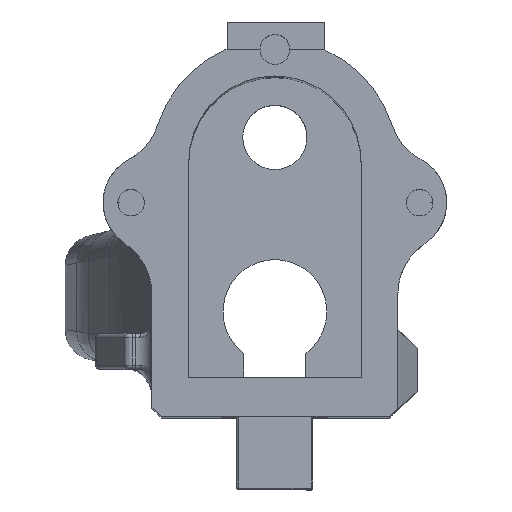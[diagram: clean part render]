
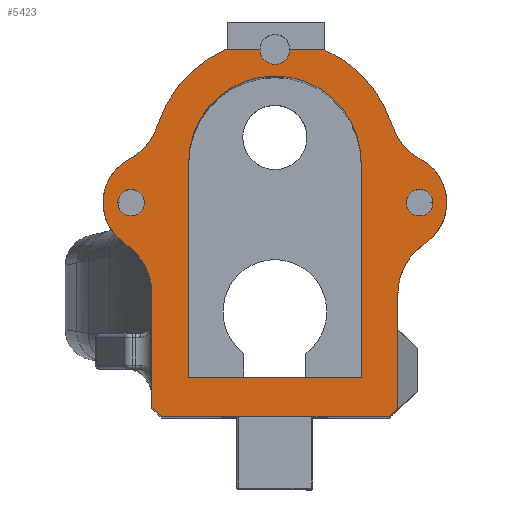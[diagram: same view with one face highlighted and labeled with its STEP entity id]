
A CAD part, top view. The second image highlights one B-rep face of the part: STEP entity #5423.
In plain terms, the highlighted planar face has unit normal (0, 0, 1).
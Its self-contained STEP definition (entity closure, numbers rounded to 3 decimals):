
#34=FACE_BOUND('',#1646,.T.);
#35=FACE_BOUND('',#1647,.T.);
#36=FACE_BOUND('',#1648,.T.);
#381=LINE('',#8278,#778);
#386=LINE('',#8334,#783);
#405=LINE('',#8480,#802);
#416=LINE('',#8525,#813);
#444=LINE('',#8599,#841);
#447=LINE('',#8604,#844);
#450=LINE('',#8622,#847);
#451=LINE('',#8631,#848);
#452=LINE('',#8634,#849);
#453=LINE('',#8638,#850);
#454=LINE('',#8639,#851);
#778=VECTOR('',#6473,1000.);
#783=VECTOR('',#6486,10.);
#802=VECTOR('',#6545,10.);
#813=VECTOR('',#6578,1000.);
#841=VECTOR('',#6622,10.);
#844=VECTOR('',#6627,10.);
#847=VECTOR('',#6648,10.);
#848=VECTOR('',#6657,1000.);
#849=VECTOR('',#6658,1000.);
#850=VECTOR('',#6661,1000.);
#851=VECTOR('',#6662,1000.);
#1294=FACE_OUTER_BOUND('',#1645,.T.);
#1645=EDGE_LOOP('',(#3883,#3884,#3885,#3886,#3887,#3888,#3889,#3890,#3891,
#3892,#3893,#3894,#3895,#3896,#3897,#3898,#3899));
#1646=EDGE_LOOP('',(#3900,#3901,#3902,#3903));
#1647=EDGE_LOOP('',(#3904));
#1648=EDGE_LOOP('',(#3905));
#2020=CIRCLE('',#5832,2.45);
#2022=CIRCLE('',#5836,10.);
#2023=CIRCLE('',#5837,8.);
#2024=CIRCLE('',#5838,10.);
#2025=CIRCLE('',#5839,20.1);
#2026=CIRCLE('',#5840,20.1);
#2027=CIRCLE('',#5841,10.);
#2028=CIRCLE('',#5842,8.);
#2029=CIRCLE('',#5843,10.);
#2030=CIRCLE('',#5844,14.1);
#2031=CIRCLE('',#5845,2.175);
#2032=CIRCLE('',#5846,2.175);
#2307=VERTEX_POINT('',#8275);
#2308=VERTEX_POINT('',#8277);
#2312=VERTEX_POINT('',#8333);
#2350=VERTEX_POINT('',#8478);
#2351=VERTEX_POINT('',#8479);
#2393=VERTEX_POINT('',#8588);
#2398=VERTEX_POINT('',#8597);
#2399=VERTEX_POINT('',#8602);
#2400=VERTEX_POINT('',#8606);
#2402=VERTEX_POINT('',#8614);
#2403=VERTEX_POINT('',#8616);
#2404=VERTEX_POINT('',#8618);
#2405=VERTEX_POINT('',#8620);
#2406=VERTEX_POINT('',#8623);
#2407=VERTEX_POINT('',#8625);
#2408=VERTEX_POINT('',#8627);
#2409=VERTEX_POINT('',#8629);
#2410=VERTEX_POINT('',#8632);
#2411=VERTEX_POINT('',#8633);
#2412=VERTEX_POINT('',#8635);
#2413=VERTEX_POINT('',#8637);
#2414=VERTEX_POINT('',#8640);
#2415=VERTEX_POINT('',#8642);
#2843=EDGE_CURVE('',#2308,#2307,#381,.T.);
#2850=EDGE_CURVE('',#2312,#2308,#386,.T.);
#2891=EDGE_CURVE('',#2350,#2351,#405,.T.);
#2912=EDGE_CURVE('',#2351,#2312,#416,.T.);
#2947=EDGE_CURVE('',#2393,#2398,#444,.T.);
#2950=EDGE_CURVE('',#2398,#2399,#447,.T.);
#2951=EDGE_CURVE('',#2400,#2393,#2020,.T.);
#2955=EDGE_CURVE('',#2307,#2402,#2022,.T.);
#2956=EDGE_CURVE('',#2403,#2402,#2023,.T.);
#2957=EDGE_CURVE('',#2403,#2404,#2024,.T.);
#2958=EDGE_CURVE('',#2404,#2405,#2025,.T.);
#2959=EDGE_CURVE('',#2405,#2400,#450,.T.);
#2960=EDGE_CURVE('',#2406,#2399,#2026,.T.);
#2961=EDGE_CURVE('',#2406,#2407,#2027,.T.);
#2962=EDGE_CURVE('',#2408,#2407,#2028,.T.);
#2963=EDGE_CURVE('',#2408,#2409,#2029,.T.);
#2964=EDGE_CURVE('',#2409,#2350,#451,.T.);
#2965=EDGE_CURVE('',#2410,#2411,#452,.T.);
#2966=EDGE_CURVE('',#2411,#2412,#2030,.T.);
#2967=EDGE_CURVE('',#2412,#2413,#453,.T.);
#2968=EDGE_CURVE('',#2413,#2410,#454,.T.);
#2969=EDGE_CURVE('',#2414,#2414,#2031,.T.);
#2970=EDGE_CURVE('',#2415,#2415,#2032,.T.);
#3883=ORIENTED_EDGE('',*,*,#2850,.T.);
#3884=ORIENTED_EDGE('',*,*,#2843,.T.);
#3885=ORIENTED_EDGE('',*,*,#2955,.T.);
#3886=ORIENTED_EDGE('',*,*,#2956,.F.);
#3887=ORIENTED_EDGE('',*,*,#2957,.T.);
#3888=ORIENTED_EDGE('',*,*,#2958,.T.);
#3889=ORIENTED_EDGE('',*,*,#2959,.T.);
#3890=ORIENTED_EDGE('',*,*,#2951,.T.);
#3891=ORIENTED_EDGE('',*,*,#2947,.T.);
#3892=ORIENTED_EDGE('',*,*,#2950,.T.);
#3893=ORIENTED_EDGE('',*,*,#2960,.F.);
#3894=ORIENTED_EDGE('',*,*,#2961,.T.);
#3895=ORIENTED_EDGE('',*,*,#2962,.F.);
#3896=ORIENTED_EDGE('',*,*,#2963,.T.);
#3897=ORIENTED_EDGE('',*,*,#2964,.T.);
#3898=ORIENTED_EDGE('',*,*,#2891,.T.);
#3899=ORIENTED_EDGE('',*,*,#2912,.T.);
#3900=ORIENTED_EDGE('',*,*,#2965,.T.);
#3901=ORIENTED_EDGE('',*,*,#2966,.T.);
#3902=ORIENTED_EDGE('',*,*,#2967,.T.);
#3903=ORIENTED_EDGE('',*,*,#2968,.T.);
#3904=ORIENTED_EDGE('',*,*,#2969,.T.);
#3905=ORIENTED_EDGE('',*,*,#2970,.T.);
#5285=PLANE('',#5835);
#5423=ADVANCED_FACE('',(#1294,#34,#35,#36),#5285,.T.);
#5832=AXIS2_PLACEMENT_3D('',#8607,#6630,#6631);
#5835=AXIS2_PLACEMENT_3D('',#8613,#6638,#6639);
#5836=AXIS2_PLACEMENT_3D('',#8615,#6640,#6641);
#5837=AXIS2_PLACEMENT_3D('',#8617,#6642,#6643);
#5838=AXIS2_PLACEMENT_3D('',#8619,#6644,#6645);
#5839=AXIS2_PLACEMENT_3D('',#8621,#6646,#6647);
#5840=AXIS2_PLACEMENT_3D('',#8624,#6649,#6650);
#5841=AXIS2_PLACEMENT_3D('',#8626,#6651,#6652);
#5842=AXIS2_PLACEMENT_3D('',#8628,#6653,#6654);
#5843=AXIS2_PLACEMENT_3D('',#8630,#6655,#6656);
#5844=AXIS2_PLACEMENT_3D('',#8636,#6659,#6660);
#5845=AXIS2_PLACEMENT_3D('',#8641,#6663,#6664);
#5846=AXIS2_PLACEMENT_3D('',#8643,#6665,#6666);
#6473=DIRECTION('',(0.,1.,0.));
#6486=DIRECTION('',(0.735,0.678,0.));
#6545=DIRECTION('',(0.735,-0.678,0.));
#6578=DIRECTION('',(1.,0.,0.));
#6622=DIRECTION('',(-1.,0.,0.));
#6627=DIRECTION('',(-1.,0.,0.));
#6630=DIRECTION('center_axis',(0.,0.,
-1.));
#6631=DIRECTION('ref_axis',(-1.,0.,0.));
#6638=DIRECTION('center_axis',(0.,0.,
1.));
#6639=DIRECTION('ref_axis',(1.,0.,0.));
#6640=DIRECTION('center_axis',(0.,0.,
-1.));
#6641=DIRECTION('ref_axis',(1.,0.,0.));
#6642=DIRECTION('center_axis',(0.,0.,
-1.));
#6643=DIRECTION('ref_axis',(1.,0.,0.));
#6644=DIRECTION('center_axis',(0.,0.,
-1.));
#6645=DIRECTION('ref_axis',(1.,0.,0.));
#6646=DIRECTION('center_axis',(0.,0.,
1.));
#6647=DIRECTION('ref_axis',(1.,0.,0.));
#6648=DIRECTION('',(-1.,0.,0.));
#6649=DIRECTION('center_axis',(0.,0.,
-1.));
#6650=DIRECTION('ref_axis',(1.,0.,0.));
#6651=DIRECTION('center_axis',(0.,0.,
-1.));
#6652=DIRECTION('ref_axis',(1.,0.,0.));
#6653=DIRECTION('center_axis',(0.,0.,
-1.));
#6654=DIRECTION('ref_axis',(1.,0.,0.));
#6655=DIRECTION('center_axis',(0.,0.,
-1.));
#6656=DIRECTION('ref_axis',(1.,0.,0.));
#6657=DIRECTION('',(0.,-1.,0.));
#6658=DIRECTION('',(0.,1.,0.));
#6659=DIRECTION('center_axis',(0.,0.,
-1.));
#6660=DIRECTION('ref_axis',(-1.,0.,0.));
#6661=DIRECTION('',(0.,-1.,0.));
#6662=DIRECTION('',(-1.,0.,0.));
#6663=DIRECTION('center_axis',(0.,0.,
-1.));
#6664=DIRECTION('ref_axis',(-1.,0.,0.));
#6665=DIRECTION('center_axis',(0.,0.,
-1.));
#6666=DIRECTION('ref_axis',(-1.,0.,0.));
#8275=CARTESIAN_POINT('',(-156.724,26.333,2.158));
#8277=CARTESIAN_POINT('',(-156.724,7.688,2.158));
#8278=CARTESIAN_POINT('',(-156.724,75.798,2.158));
#8333=CARTESIAN_POINT('',(-158.161,6.363,2.158));
#8334=CARTESIAN_POINT('',(-138.035,24.927,2.158));
#8478=CARTESIAN_POINT('',(-196.924,7.866,2.158));
#8479=CARTESIAN_POINT('',(-195.294,6.363,2.158));
#8480=CARTESIAN_POINT('',(-202.177,12.711,2.158));
#8525=CARTESIAN_POINT('',(-156.724,6.363,2.158));
#8588=CARTESIAN_POINT('',(-179.274,66.352,2.158));
#8597=CARTESIAN_POINT('',(-184.649,66.352,2.158));
#8599=CARTESIAN_POINT('',(-162.774,66.352,2.158));
#8602=CARTESIAN_POINT('',(-184.824,66.352,2.158));
#8604=CARTESIAN_POINT('',(-162.774,66.352,2.158));
#8606=CARTESIAN_POINT('',(-174.374,66.352,2.158));
#8607=CARTESIAN_POINT('Origin',(-176.824,66.352,2.158));
#8613=CARTESIAN_POINT('Origin',(-156.724,75.798,2.158));
#8614=CARTESIAN_POINT('',(-152.28,34.648,2.158));
#8615=CARTESIAN_POINT('Origin',(-146.724,26.333,2.158));
#8616=CARTESIAN_POINT('',(-152.924,48.34,2.158));
#8617=CARTESIAN_POINT('Origin',(-156.724,41.3,2.158));
#8618=CARTESIAN_POINT('',(-157.692,54.074,2.158));
#8619=CARTESIAN_POINT('Origin',(-148.173,57.139,2.158));
#8620=CARTESIAN_POINT('',(-168.824,66.352,2.158));
#8621=CARTESIAN_POINT('Origin',(-176.824,47.913,2.158));
#8622=CARTESIAN_POINT('',(-162.774,66.352,2.158));
#8623=CARTESIAN_POINT('',(-195.957,54.074,2.158));
#8624=CARTESIAN_POINT('Origin',(-176.824,47.913,2.158));
#8625=CARTESIAN_POINT('',(-200.725,48.34,2.158));
#8626=CARTESIAN_POINT('Origin',(-205.475,57.139,2.158));
#8627=CARTESIAN_POINT('',(-201.369,34.648,2.158));
#8628=CARTESIAN_POINT('Origin',(-196.924,41.3,2.158));
#8629=CARTESIAN_POINT('',(-196.924,26.333,2.158));
#8630=CARTESIAN_POINT('Origin',(-206.924,26.333,2.158));
#8631=CARTESIAN_POINT('',(-196.924,75.798,2.158));
#8632=CARTESIAN_POINT('',(-190.924,12.713,2.158));
#8633=CARTESIAN_POINT('',(-190.924,47.913,2.158));
#8634=CARTESIAN_POINT('',(-190.924,75.798,2.158));
#8635=CARTESIAN_POINT('',(-162.724,47.913,2.158));
#8636=CARTESIAN_POINT('Origin',(-176.824,47.913,2.158));
#8637=CARTESIAN_POINT('',(-162.724,12.713,2.158));
#8638=CARTESIAN_POINT('',(-162.724,75.798,2.158));
#8639=CARTESIAN_POINT('',(-156.724,12.713,2.158));
#8640=CARTESIAN_POINT('',(-198.149,41.3,2.158));
#8641=CARTESIAN_POINT('Origin',(-200.324,41.3,2.158));
#8642=CARTESIAN_POINT('',(-151.,41.3,2.158));
#8643=CARTESIAN_POINT('Origin',(-153.175,41.3,2.158));
